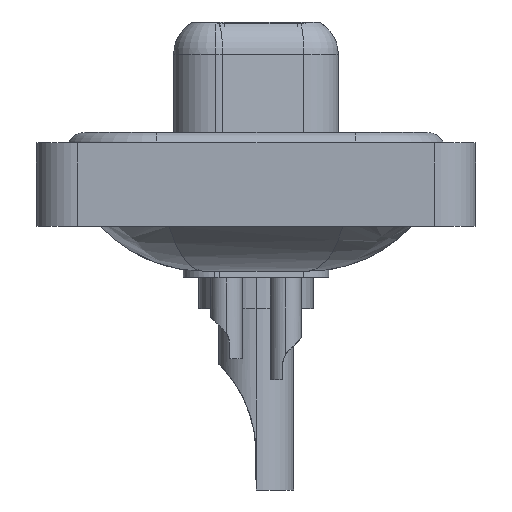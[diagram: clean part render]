
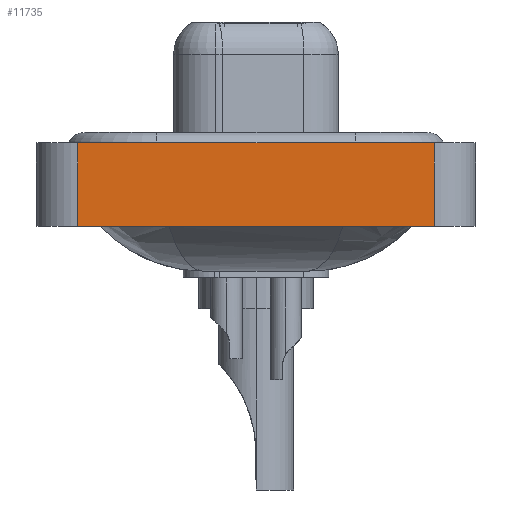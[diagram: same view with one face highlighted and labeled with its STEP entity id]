
A CAD part, left-side view. The second image highlights one B-rep face of the part: STEP entity #11735.
In plain terms, the highlighted planar face has unit normal (-1, 0, 0).
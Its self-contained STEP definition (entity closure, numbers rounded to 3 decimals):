
#87 = EDGE_CURVE ( 'NONE', #14703, #10097, #18491, .T. ) ;
#235 = FACE_OUTER_BOUND ( 'NONE', #10008, .T. ) ;
#1428 = CARTESIAN_POINT ( 'NONE',  ( -7.35, -8.55, -3.6 ) ) ;
#2736 = VECTOR ( 'NONE', #4469, 1000. ) ;
#4469 = DIRECTION ( 'NONE',  ( 0., -1., 0. ) ) ;
#4524 = CARTESIAN_POINT ( 'NONE',  ( -7.35, -8.55, -3.6 ) ) ;
#5895 = CARTESIAN_POINT ( 'NONE',  ( -7.35, -8.55, 0.4 ) ) ;
#7192 = VERTEX_POINT ( 'NONE', #11149 ) ;
#7651 = LINE ( 'NONE', #15919, #13256 ) ;
#7715 = LINE ( 'NONE', #23785, #22254 ) ;
#8346 = CARTESIAN_POINT ( 'NONE',  ( -7.35, -8.55, -3.6 ) ) ;
#9584 = DIRECTION ( 'NONE',  ( 0., 0., 1. ) ) ;
#10008 = EDGE_LOOP ( 'NONE', ( #10482, #15119, #19863, #14480 ) ) ;
#10097 = VERTEX_POINT ( 'NONE', #16960 ) ;
#10482 = ORIENTED_EDGE ( 'NONE', *, *, #22769, .T. ) ;
#10878 = AXIS2_PLACEMENT_3D ( 'NONE', #4524, #22449, #16534 ) ;
#11149 = CARTESIAN_POINT ( 'NONE',  ( -7.35, 8.55, 0.4 ) ) ;
#11188 = VECTOR ( 'NONE', #9584, 1000. ) ;
#11735 = ADVANCED_FACE ( 'NONE', ( #235 ), #18675, .T. ) ;
#13256 = VECTOR ( 'NONE', #13663, 1000. ) ;
#13663 = DIRECTION ( 'NONE',  ( 0., 0., 1. ) ) ;
#13796 = CARTESIAN_POINT ( 'NONE',  ( -7.35, 8.55, -3.6 ) ) ;
#13983 = LINE ( 'NONE', #1428, #11188 ) ;
#14480 = ORIENTED_EDGE ( 'NONE', *, *, #87, .T. ) ;
#14703 = VERTEX_POINT ( 'NONE', #13796 ) ;
#15119 = ORIENTED_EDGE ( 'NONE', *, *, #25405, .F. ) ;
#15919 = CARTESIAN_POINT ( 'NONE',  ( -7.35, 8.55, -3.6 ) ) ;
#16534 = DIRECTION ( 'NONE',  ( 0., 0., 1. ) ) ;
#16960 = CARTESIAN_POINT ( 'NONE',  ( -7.35, -8.55, -3.6 ) ) ;
#18491 = LINE ( 'NONE', #8346, #2736 ) ;
#18675 = PLANE ( 'NONE',  #10878 ) ;
#19863 = ORIENTED_EDGE ( 'NONE', *, *, #24965, .F. ) ;
#20702 = VERTEX_POINT ( 'NONE', #5895 ) ;
#22254 = VECTOR ( 'NONE', #23911, 1000. ) ;
#22449 = DIRECTION ( 'NONE',  ( -1., 0., 0. ) ) ;
#22769 = EDGE_CURVE ( 'NONE', #10097, #20702, #13983, .T. ) ;
#23785 = CARTESIAN_POINT ( 'NONE',  ( -7.35, -8.55, 0.4 ) ) ;
#23911 = DIRECTION ( 'NONE',  ( 0., -1., 0. ) ) ;
#24965 = EDGE_CURVE ( 'NONE', #14703, #7192, #7651, .T. ) ;
#25405 = EDGE_CURVE ( 'NONE', #7192, #20702, #7715, .T. ) ;
